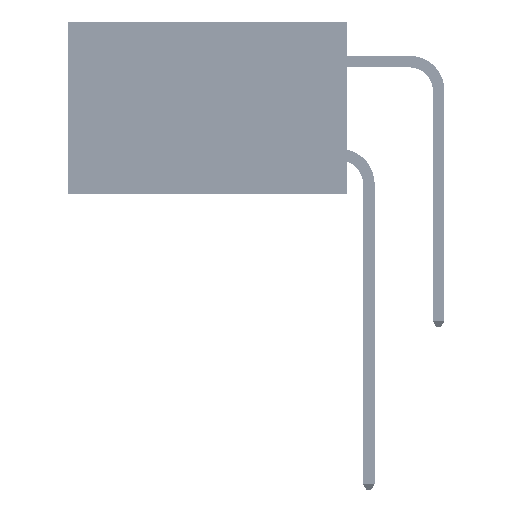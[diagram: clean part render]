
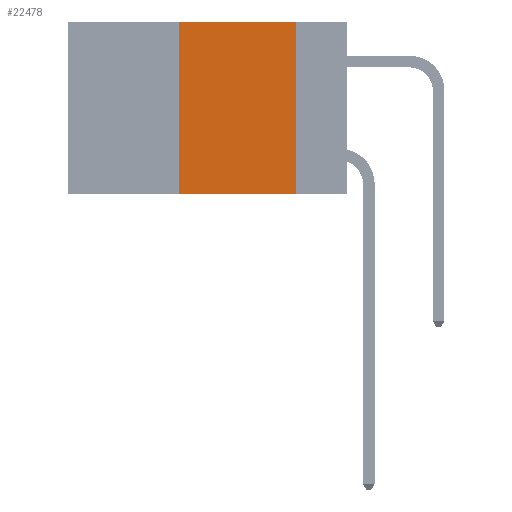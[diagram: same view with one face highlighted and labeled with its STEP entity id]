
A CAD part, left-side view. The second image highlights one B-rep face of the part: STEP entity #22478.
In plain terms, the highlighted planar face has unit normal (-1, 0, 0).
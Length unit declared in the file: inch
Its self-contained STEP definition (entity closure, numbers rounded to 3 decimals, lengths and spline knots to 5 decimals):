
#917 = CARTESIAN_POINT ( 'NONE',  ( 0., 0.36, 0. ) ) ;
#5072 = DIRECTION ( 'NONE',  ( 0., 0., 1. ) ) ;
#5649 = DIRECTION ( 'NONE',  ( 0., -1., 0. ) ) ;
#6335 = ORIENTED_EDGE ( 'NONE', *, *, #24257, .F. ) ;
#8202 = EDGE_CURVE ( 'NONE', #34456, #49731, #26518, .T. ) ;
#8900 = DIRECTION ( 'NONE',  ( 0., -1., 0. ) ) ;
#9007 = LINE ( 'NONE', #44640, #28978 ) ;
#9910 = CARTESIAN_POINT ( 'NONE',  ( 0., 0.6, 0. ) ) ;
#10175 = LINE ( 'NONE', #25609, #39346 ) ;
#13963 = DIRECTION ( 'NONE',  ( 0., 0., -1. ) ) ;
#17271 = EDGE_CURVE ( 'NONE', #34456, #46238, #10175, .T. ) ;
#17538 = LINE ( 'NONE', #20226, #26857 ) ;
#18411 = ORIENTED_EDGE ( 'NONE', *, *, #17271, .T. ) ;
#20226 = CARTESIAN_POINT ( 'NONE',  ( 0., 0.11, 0. ) ) ;
#20999 = EDGE_CURVE ( 'NONE', #49731, #35838, #9007, .T. ) ;
#22478 = ADVANCED_FACE ( 'NONE', ( #34404 ), #45443, .F. ) ;
#24257 = EDGE_CURVE ( 'NONE', #35838, #46238, #17538, .T. ) ;
#25176 = ORIENTED_EDGE ( 'NONE', *, *, #8202, .F. ) ;
#25609 = CARTESIAN_POINT ( 'NONE',  ( 0., 0.6, -0.37 ) ) ;
#26518 = LINE ( 'NONE', #917, #46263 ) ;
#26857 = VECTOR ( 'NONE', #39767, 39.37008 ) ;
#27747 = CARTESIAN_POINT ( 'NONE',  ( 0., 0.11, -0.37 ) ) ;
#28978 = VECTOR ( 'NONE', #8900, 39.37008 ) ;
#31854 = CARTESIAN_POINT ( 'NONE',  ( 0., 0.36, 0. ) ) ;
#34404 = FACE_OUTER_BOUND ( 'NONE', #35129, .T. ) ;
#34456 = VERTEX_POINT ( 'NONE', #48496 ) ;
#35129 = EDGE_LOOP ( 'NONE', ( #6335, #44317, #25176, #18411 ) ) ;
#35838 = VERTEX_POINT ( 'NONE', #37439 ) ;
#37439 = CARTESIAN_POINT ( 'NONE',  ( 0., 0.11, 0. ) ) ;
#37699 = DIRECTION ( 'NONE',  ( 1., 0., 0. ) ) ;
#39346 = VECTOR ( 'NONE', #5649, 39.37008 ) ;
#39767 = DIRECTION ( 'NONE',  ( 0., 0., -1. ) ) ;
#44317 = ORIENTED_EDGE ( 'NONE', *, *, #20999, .F. ) ;
#44640 = CARTESIAN_POINT ( 'NONE',  ( 0., 0.6, 0. ) ) ;
#45443 = PLANE ( 'NONE',  #47788 ) ;
#46238 = VERTEX_POINT ( 'NONE', #27747 ) ;
#46263 = VECTOR ( 'NONE', #5072, 39.37008 ) ;
#47788 = AXIS2_PLACEMENT_3D ( 'NONE', #9910, #37699, #13963 ) ;
#48496 = CARTESIAN_POINT ( 'NONE',  ( 0., 0.36, -0.37 ) ) ;
#49731 = VERTEX_POINT ( 'NONE', #31854 ) ;
